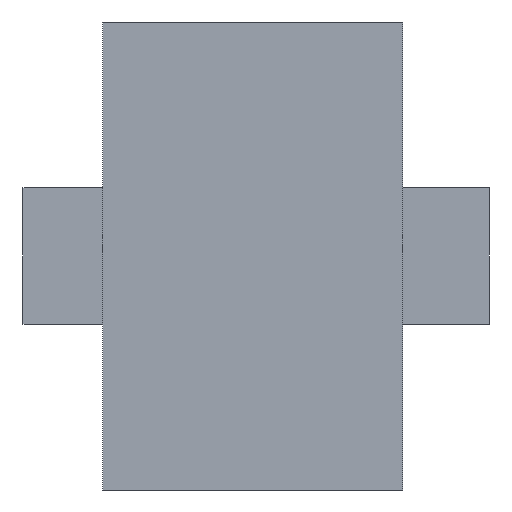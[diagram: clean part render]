
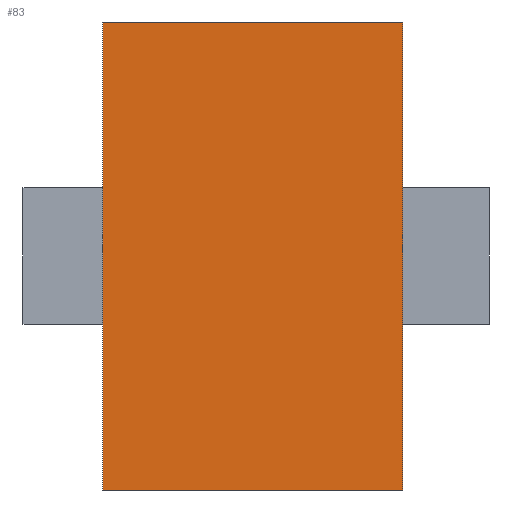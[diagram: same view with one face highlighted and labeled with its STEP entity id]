
A CAD part, front view. The second image highlights one B-rep face of the part: STEP entity #83.
In plain terms, the highlighted planar face has unit normal (0, -1, 0).
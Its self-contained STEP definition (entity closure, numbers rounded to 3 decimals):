
#5 = ORIENTED_EDGE ( 'NONE', *, *, #397, .F. ) ;
#12 = CARTESIAN_POINT ( 'NONE',  ( 71.045, 8.634, 0. ) ) ;
#13 = VECTOR ( 'NONE', #143, 1000. ) ;
#38 = LINE ( 'NONE', #234, #101 ) ;
#45 = DIRECTION ( 'NONE',  ( 1., 0., 0. ) ) ;
#60 = VERTEX_POINT ( 'NONE', #69 ) ;
#62 = DIRECTION ( 'NONE',  ( 0., -1., 0. ) ) ;
#69 = CARTESIAN_POINT ( 'NONE',  ( 71.045, 8.634, -5.944 ) ) ;
#79 = DIRECTION ( 'NONE',  ( 0., 0., 1. ) ) ;
#81 = CARTESIAN_POINT ( 'NONE',  ( 71.045, 8.634, 0. ) ) ;
#83 = ADVANCED_FACE ( 'NONE', ( #316 ), #195, .T. ) ;
#85 = VECTOR ( 'NONE', #146, 1000. ) ;
#89 = ORIENTED_EDGE ( 'NONE', *, *, #395, .F. ) ;
#94 = LINE ( 'NONE', #81, #373 ) ;
#101 = VECTOR ( 'NONE', #214, 1000. ) ;
#122 = ORIENTED_EDGE ( 'NONE', *, *, #383, .F. ) ;
#133 = CARTESIAN_POINT ( 'NONE',  ( 71.045, 8.634, 5.944 ) ) ;
#143 = DIRECTION ( 'NONE',  ( 0., 0., 1. ) ) ;
#146 = DIRECTION ( 'NONE',  ( 1., 0., 0. ) ) ;
#164 = CARTESIAN_POINT ( 'NONE',  ( 78.665, 8.634, 0. ) ) ;
#165 = CARTESIAN_POINT ( 'NONE',  ( 78.665, 8.634, 5.944 ) ) ;
#172 = VERTEX_POINT ( 'NONE', #398 ) ;
#195 = PLANE ( 'NONE',  #352 ) ;
#214 = DIRECTION ( 'NONE',  ( -1., 0., 0. ) ) ;
#217 = ORIENTED_EDGE ( 'NONE', *, *, #390, .T. ) ;
#234 = CARTESIAN_POINT ( 'NONE',  ( 71.045, 8.634, -5.944 ) ) ;
#282 = LINE ( 'NONE', #164, #13 ) ;
#316 = FACE_OUTER_BOUND ( 'NONE', #476, .T. ) ;
#352 = AXIS2_PLACEMENT_3D ( 'NONE', #12, #62, #45 ) ;
#369 = CARTESIAN_POINT ( 'NONE',  ( 78.665, 8.634, -5.944 ) ) ;
#373 = VECTOR ( 'NONE', #79, 1000. ) ;
#383 = EDGE_CURVE ( 'NONE', #457, #60, #38, .T. ) ;
#384 = LINE ( 'NONE', #133, #85 ) ;
#390 = EDGE_CURVE ( 'NONE', #457, #428, #282, .T. ) ;
#395 = EDGE_CURVE ( 'NONE', #172, #428, #384, .T. ) ;
#397 = EDGE_CURVE ( 'NONE', #60, #172, #94, .T. ) ;
#398 = CARTESIAN_POINT ( 'NONE',  ( 71.045, 8.634, 5.944 ) ) ;
#428 = VERTEX_POINT ( 'NONE', #165 ) ;
#457 = VERTEX_POINT ( 'NONE', #369 ) ;
#476 = EDGE_LOOP ( 'NONE', ( #217, #89, #5, #122 ) ) ;
